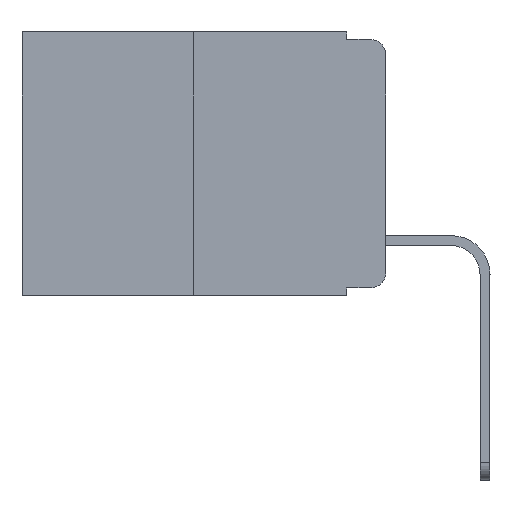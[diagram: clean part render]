
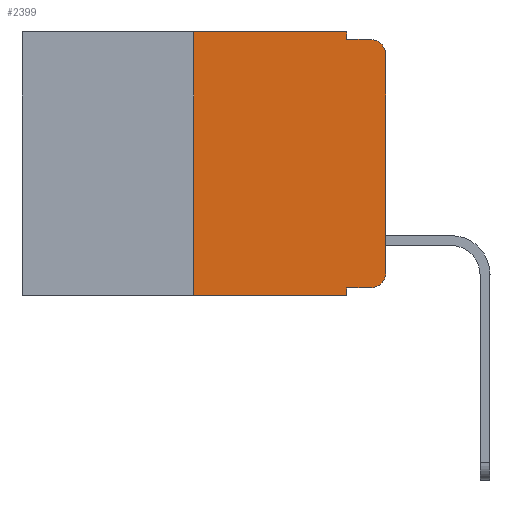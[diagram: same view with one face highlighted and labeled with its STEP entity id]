
A CAD part, left-side view. The second image highlights one B-rep face of the part: STEP entity #2399.
In plain terms, the highlighted planar face has unit normal (-1, 0, 0).
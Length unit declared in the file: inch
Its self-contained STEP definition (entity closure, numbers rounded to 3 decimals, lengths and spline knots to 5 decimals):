
#228 = VERTEX_POINT ( 'NONE', #16663 ) ;
#935 = CARTESIAN_POINT ( 'NONE',  ( 0., 0.051, 0. ) ) ;
#1318 = CARTESIAN_POINT ( 'NONE',  ( 0., 0., -0.03 ) ) ;
#1861 = ORIENTED_EDGE ( 'NONE', *, *, #16309, .T. ) ;
#2270 = AXIS2_PLACEMENT_3D ( 'NONE', #14263, #3214, #21595 ) ;
#2399 = ADVANCED_FACE ( 'NONE', ( #3406 ), #3652, .F. ) ;
#2538 = VERTEX_POINT ( 'NONE', #9033 ) ;
#2867 = ORIENTED_EDGE ( 'NONE', *, *, #3055, .T. ) ;
#3055 = EDGE_CURVE ( 'NONE', #9055, #7083, #13323, .T. ) ;
#3214 = DIRECTION ( 'NONE',  ( -1., 0., 0. ) ) ;
#3289 = EDGE_CURVE ( 'NONE', #10261, #12435, #21864, .T. ) ;
#3406 = FACE_OUTER_BOUND ( 'NONE', #11547, .T. ) ;
#3565 = VERTEX_POINT ( 'NONE', #16935 ) ;
#3585 = EDGE_CURVE ( 'NONE', #22317, #3565, #15041, .T. ) ;
#3652 = PLANE ( 'NONE',  #19331 ) ;
#3757 = ORIENTED_EDGE ( 'NONE', *, *, #21505, .T. ) ;
#3998 = CARTESIAN_POINT ( 'NONE',  ( 0., 0.02, -0.03 ) ) ;
#5673 = DIRECTION ( 'NONE',  ( 0., 0., -1. ) ) ;
#5820 = DIRECTION ( 'NONE',  ( 0., -1., 0. ) ) ;
#6047 = VERTEX_POINT ( 'NONE', #16071 ) ;
#6177 = VECTOR ( 'NONE', #16843, 39.37008 ) ;
#6366 = LINE ( 'NONE', #19654, #15443 ) ;
#6811 = EDGE_CURVE ( 'NONE', #3565, #6047, #9230, .T. ) ;
#6993 = EDGE_CURVE ( 'NONE', #6047, #7083, #6366, .T. ) ;
#7083 = VERTEX_POINT ( 'NONE', #14912 ) ;
#7291 = ORIENTED_EDGE ( 'NONE', *, *, #6811, .F. ) ;
#7474 = CARTESIAN_POINT ( 'NONE',  ( 0., 0.051, -0.333 ) ) ;
#7559 = CARTESIAN_POINT ( 'NONE',  ( 0., 0.25, 0. ) ) ;
#7659 = DIRECTION ( 'NONE',  ( 0., -1., 0. ) ) ;
#8588 = DIRECTION ( 'NONE',  ( 0., 0., -1. ) ) ;
#8888 = LINE ( 'NONE', #18278, #17404 ) ;
#9003 = DIRECTION ( 'NONE',  ( 1., 0., 0. ) ) ;
#9033 = CARTESIAN_POINT ( 'NONE',  ( 0., 0.25, -0.343 ) ) ;
#9055 = VERTEX_POINT ( 'NONE', #1318 ) ;
#9230 = LINE ( 'NONE', #935, #21428 ) ;
#10261 = VERTEX_POINT ( 'NONE', #12440 ) ;
#10511 = EDGE_CURVE ( 'NONE', #2538, #22317, #20680, .T. ) ;
#10602 = LINE ( 'NONE', #23270, #18592 ) ;
#11001 = CARTESIAN_POINT ( 'NONE',  ( 0., 0.25, 0. ) ) ;
#11547 = EDGE_LOOP ( 'NONE', ( #1861, #2867, #21345, #7291, #23251, #21175, #18135, #19976, #22440, #3757 ) ) ;
#12403 = DIRECTION ( 'NONE',  ( 0., 0., 1. ) ) ;
#12435 = VERTEX_POINT ( 'NONE', #19591 ) ;
#12440 = CARTESIAN_POINT ( 'NONE',  ( 0., 0.051, -0.333 ) ) ;
#12687 = LINE ( 'NONE', #7474, #18448 ) ;
#12893 = EDGE_CURVE ( 'NONE', #2538, #12435, #8888, .T. ) ;
#12956 = DIRECTION ( 'NONE',  ( -1., 0., 0. ) ) ;
#13323 = CIRCLE ( 'NONE', #15953, 0.02 ) ;
#13800 = DIRECTION ( 'NONE',  ( 0., -1., 0. ) ) ;
#13844 = VERTEX_POINT ( 'NONE', #22001 ) ;
#13997 = DIRECTION ( 'NONE',  ( 0., 0., -1. ) ) ;
#14263 = CARTESIAN_POINT ( 'NONE',  ( 0., 0.02, -0.313 ) ) ;
#14321 = EDGE_CURVE ( 'NONE', #10261, #228, #12687, .T. ) ;
#14912 = CARTESIAN_POINT ( 'NONE',  ( 0., 0.02, -0.01 ) ) ;
#15041 = LINE ( 'NONE', #20473, #15858 ) ;
#15443 = VECTOR ( 'NONE', #13800, 39.37008 ) ;
#15858 = VECTOR ( 'NONE', #7659, 39.37008 ) ;
#15953 = AXIS2_PLACEMENT_3D ( 'NONE', #3998, #12956, #18485 ) ;
#16071 = CARTESIAN_POINT ( 'NONE',  ( 0., 0.051, -0.01 ) ) ;
#16309 = EDGE_CURVE ( 'NONE', #13844, #9055, #10602, .T. ) ;
#16454 = CARTESIAN_POINT ( 'NONE',  ( 0., 0.473, 0. ) ) ;
#16513 = CIRCLE ( 'NONE', #2270, 0.02 ) ;
#16663 = CARTESIAN_POINT ( 'NONE',  ( 0., 0.02, -0.333 ) ) ;
#16843 = DIRECTION ( 'NONE',  ( 0., 0., 1. ) ) ;
#16935 = CARTESIAN_POINT ( 'NONE',  ( 0., 0.051, 0. ) ) ;
#17306 = VECTOR ( 'NONE', #8588, 39.37008 ) ;
#17404 = VECTOR ( 'NONE', #18029, 39.37008 ) ;
#18029 = DIRECTION ( 'NONE',  ( 0., -1., 0. ) ) ;
#18135 = ORIENTED_EDGE ( 'NONE', *, *, #12893, .T. ) ;
#18278 = CARTESIAN_POINT ( 'NONE',  ( 0., 0.473, -0.343 ) ) ;
#18448 = VECTOR ( 'NONE', #5820, 39.37008 ) ;
#18485 = DIRECTION ( 'NONE',  ( 0., 0., -1. ) ) ;
#18592 = VECTOR ( 'NONE', #12403, 39.37008 ) ;
#19331 = AXIS2_PLACEMENT_3D ( 'NONE', #16454, #9003, #5673 ) ;
#19507 = CARTESIAN_POINT ( 'NONE',  ( 0., 0.051, 0. ) ) ;
#19591 = CARTESIAN_POINT ( 'NONE',  ( 0., 0.051, -0.343 ) ) ;
#19654 = CARTESIAN_POINT ( 'NONE',  ( 0., 0.051, -0.01 ) ) ;
#19976 = ORIENTED_EDGE ( 'NONE', *, *, #3289, .F. ) ;
#20473 = CARTESIAN_POINT ( 'NONE',  ( 0., 0.473, 0. ) ) ;
#20680 = LINE ( 'NONE', #7559, #6177 ) ;
#21175 = ORIENTED_EDGE ( 'NONE', *, *, #10511, .F. ) ;
#21345 = ORIENTED_EDGE ( 'NONE', *, *, #6993, .F. ) ;
#21428 = VECTOR ( 'NONE', #13997, 39.37008 ) ;
#21505 = EDGE_CURVE ( 'NONE', #228, #13844, #16513, .T. ) ;
#21595 = DIRECTION ( 'NONE',  ( 0., 0., -1. ) ) ;
#21864 = LINE ( 'NONE', #19507, #17306 ) ;
#22001 = CARTESIAN_POINT ( 'NONE',  ( 0., 0., -0.313 ) ) ;
#22317 = VERTEX_POINT ( 'NONE', #11001 ) ;
#22440 = ORIENTED_EDGE ( 'NONE', *, *, #14321, .T. ) ;
#23251 = ORIENTED_EDGE ( 'NONE', *, *, #3585, .F. ) ;
#23270 = CARTESIAN_POINT ( 'NONE',  ( 0., 0., 0. ) ) ;
